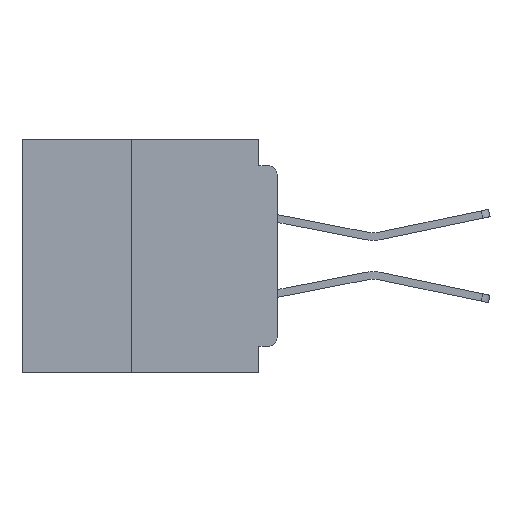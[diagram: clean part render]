
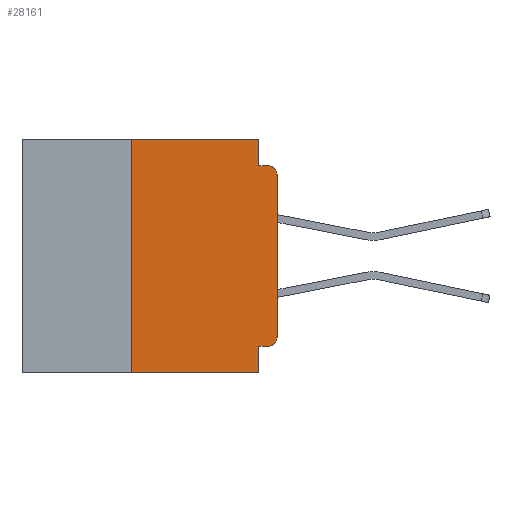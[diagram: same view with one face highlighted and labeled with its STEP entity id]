
A CAD part, left-side view. The second image highlights one B-rep face of the part: STEP entity #28161.
In plain terms, the highlighted planar face has unit normal (-1, 0, 0).
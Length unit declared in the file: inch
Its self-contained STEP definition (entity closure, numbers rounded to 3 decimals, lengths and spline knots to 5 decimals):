
#1152 = AXIS2_PLACEMENT_3D ( 'NONE', #9055, #37229, #13175 ) ;
#1810 = VECTOR ( 'NONE', #38327, 39.37008 ) ;
#3036 = PLANE ( 'NONE',  #42962 ) ;
#3450 = CARTESIAN_POINT ( 'NONE',  ( 0., 0.031, 0. ) ) ;
#4617 = ORIENTED_EDGE ( 'NONE', *, *, #29067, .F. ) ;
#6388 = EDGE_CURVE ( 'NONE', #11730, #7666, #33943, .T. ) ;
#6428 = CARTESIAN_POINT ( 'NONE',  ( 0., 0.015, -0.06 ) ) ;
#7031 = DIRECTION ( 'NONE',  ( 0., -1., 0. ) ) ;
#7214 = VECTOR ( 'NONE', #14709, 39.37008 ) ;
#7666 = VERTEX_POINT ( 'NONE', #49822 ) ;
#8297 = LINE ( 'NONE', #46679, #49728 ) ;
#9055 = CARTESIAN_POINT ( 'NONE',  ( 0., 0.015, -0.34 ) ) ;
#10009 = EDGE_CURVE ( 'NONE', #16631, #20322, #42372, .T. ) ;
#10462 = DIRECTION ( 'NONE',  ( 0., 0., 1. ) ) ;
#10516 = DIRECTION ( 'NONE',  ( 0., 0., -1. ) ) ;
#10628 = CARTESIAN_POINT ( 'NONE',  ( 0., 0., -0.355 ) ) ;
#11210 = CARTESIAN_POINT ( 'NONE',  ( 0., 0.437, 0. ) ) ;
#11322 = ORIENTED_EDGE ( 'NONE', *, *, #17192, .F. ) ;
#11730 = VERTEX_POINT ( 'NONE', #32645 ) ;
#12891 = CARTESIAN_POINT ( 'NONE',  ( 0., 0.031, -0.4 ) ) ;
#13118 = CARTESIAN_POINT ( 'NONE',  ( 0., 0.031, 0. ) ) ;
#13175 = DIRECTION ( 'NONE',  ( 0., 0., -1. ) ) ;
#13880 = LINE ( 'NONE', #44800, #1810 ) ;
#14223 = LINE ( 'NONE', #14527, #44941 ) ;
#14296 = EDGE_CURVE ( 'NONE', #19391, #16631, #13880, .T. ) ;
#14527 = CARTESIAN_POINT ( 'NONE',  ( 0., 0.25, -0.4 ) ) ;
#14709 = DIRECTION ( 'NONE',  ( 0., 1., 0. ) ) ;
#15252 = DIRECTION ( 'NONE',  ( 0., 0., -1. ) ) ;
#15323 = ORIENTED_EDGE ( 'NONE', *, *, #44863, .F. ) ;
#15967 = ORIENTED_EDGE ( 'NONE', *, *, #23770, .F. ) ;
#16631 = VERTEX_POINT ( 'NONE', #35403 ) ;
#17192 = EDGE_CURVE ( 'NONE', #22354, #20322, #8297, .T. ) ;
#18822 = EDGE_CURVE ( 'NONE', #37340, #50357, #46466, .T. ) ;
#19391 = VERTEX_POINT ( 'NONE', #34098 ) ;
#19738 = EDGE_CURVE ( 'NONE', #39521, #19391, #33231, .T. ) ;
#20156 = LINE ( 'NONE', #13118, #50807 ) ;
#20322 = VERTEX_POINT ( 'NONE', #36195 ) ;
#22354 = VERTEX_POINT ( 'NONE', #25821 ) ;
#23249 = VECTOR ( 'NONE', #41948, 39.37008 ) ;
#23770 = EDGE_CURVE ( 'NONE', #34235, #7666, #39184, .T. ) ;
#25718 = EDGE_LOOP ( 'NONE', ( #32073, #28949, #11322, #15323, #28532, #51005, #32335, #15967, #4617, #27320 ) ) ;
#25821 = CARTESIAN_POINT ( 'NONE',  ( 0., 0.031, -0.045 ) ) ;
#27320 = ORIENTED_EDGE ( 'NONE', *, *, #19738, .T. ) ;
#27968 = AXIS2_PLACEMENT_3D ( 'NONE', #6428, #34603, #10516 ) ;
#28161 = ADVANCED_FACE ( 'NONE', ( #41876 ), #3036, .F. ) ;
#28476 = VECTOR ( 'NONE', #40625, 39.37008 ) ;
#28532 = ORIENTED_EDGE ( 'NONE', *, *, #18822, .F. ) ;
#28949 = ORIENTED_EDGE ( 'NONE', *, *, #10009, .T. ) ;
#29067 = EDGE_CURVE ( 'NONE', #39521, #34235, #39322, .T. ) ;
#30582 = CARTESIAN_POINT ( 'NONE',  ( 0., 0.015, -0.355 ) ) ;
#31157 = CARTESIAN_POINT ( 'NONE',  ( 0., 0.437, 0. ) ) ;
#32073 = ORIENTED_EDGE ( 'NONE', *, *, #14296, .T. ) ;
#32204 = CARTESIAN_POINT ( 'NONE',  ( 0., 0.25, 0. ) ) ;
#32335 = ORIENTED_EDGE ( 'NONE', *, *, #6388, .T. ) ;
#32645 = CARTESIAN_POINT ( 'NONE',  ( 0., 0.25, -0.4 ) ) ;
#33231 = CIRCLE ( 'NONE', #1152, 0.015 ) ;
#33943 = LINE ( 'NONE', #37771, #23249 ) ;
#34098 = CARTESIAN_POINT ( 'NONE',  ( 0., 0., -0.34 ) ) ;
#34235 = VERTEX_POINT ( 'NONE', #47506 ) ;
#34603 = DIRECTION ( 'NONE',  ( -1., 0., 0. ) ) ;
#35403 = CARTESIAN_POINT ( 'NONE',  ( 0., 0., -0.06 ) ) ;
#35868 = VECTOR ( 'NONE', #7031, 39.37008 ) ;
#36195 = CARTESIAN_POINT ( 'NONE',  ( 0., 0.015, -0.045 ) ) ;
#37229 = DIRECTION ( 'NONE',  ( -1., 0., 0. ) ) ;
#37340 = VERTEX_POINT ( 'NONE', #32204 ) ;
#37771 = CARTESIAN_POINT ( 'NONE',  ( 0., 0.437, -0.4 ) ) ;
#38302 = EDGE_CURVE ( 'NONE', #11730, #37340, #14223, .T. ) ;
#38327 = DIRECTION ( 'NONE',  ( 0., 0., 1. ) ) ;
#38663 = DIRECTION ( 'NONE',  ( 0., -1., 0. ) ) ;
#39184 = LINE ( 'NONE', #12891, #28476 ) ;
#39322 = LINE ( 'NONE', #10628, #7214 ) ;
#39338 = DIRECTION ( 'NONE',  ( 1., 0., 0. ) ) ;
#39521 = VERTEX_POINT ( 'NONE', #30582 ) ;
#40625 = DIRECTION ( 'NONE',  ( 0., 0., -1. ) ) ;
#41876 = FACE_OUTER_BOUND ( 'NONE', #25718, .T. ) ;
#41948 = DIRECTION ( 'NONE',  ( 0., -1., 0. ) ) ;
#42372 = CIRCLE ( 'NONE', #27968, 0.015 ) ;
#42962 = AXIS2_PLACEMENT_3D ( 'NONE', #11210, #39338, #15252 ) ;
#44800 = CARTESIAN_POINT ( 'NONE',  ( 0., 0., 0. ) ) ;
#44863 = EDGE_CURVE ( 'NONE', #50357, #22354, #20156, .T. ) ;
#44941 = VECTOR ( 'NONE', #10462, 39.37008 ) ;
#45183 = DIRECTION ( 'NONE',  ( 0., 0., -1. ) ) ;
#46466 = LINE ( 'NONE', #31157, #35868 ) ;
#46679 = CARTESIAN_POINT ( 'NONE',  ( 0., 0., -0.045 ) ) ;
#47506 = CARTESIAN_POINT ( 'NONE',  ( 0., 0.031, -0.355 ) ) ;
#49728 = VECTOR ( 'NONE', #38663, 39.37008 ) ;
#49822 = CARTESIAN_POINT ( 'NONE',  ( 0., 0.031, -0.4 ) ) ;
#50357 = VERTEX_POINT ( 'NONE', #3450 ) ;
#50807 = VECTOR ( 'NONE', #45183, 39.37008 ) ;
#51005 = ORIENTED_EDGE ( 'NONE', *, *, #38302, .F. ) ;
